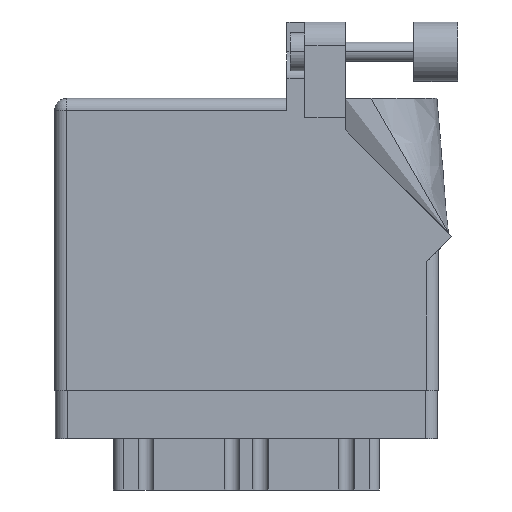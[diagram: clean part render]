
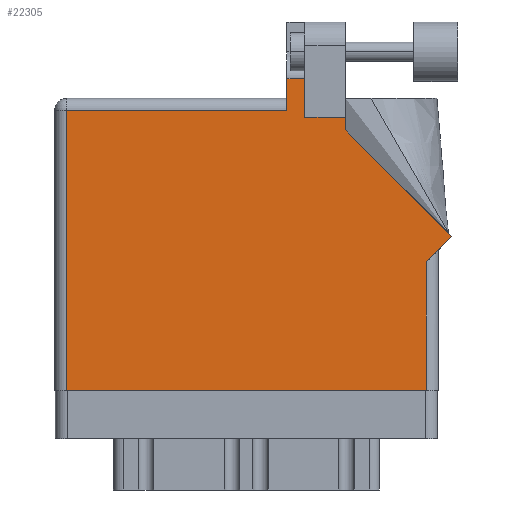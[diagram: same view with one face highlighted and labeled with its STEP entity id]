
A CAD part, front view. The second image highlights one B-rep face of the part: STEP entity #22305.
In plain terms, the highlighted face is planar.
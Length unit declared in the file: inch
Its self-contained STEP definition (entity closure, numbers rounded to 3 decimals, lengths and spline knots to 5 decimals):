
#768 = VECTOR ( 'NONE', #8616, 39.37008 ) ;
#2090 = VERTEX_POINT ( 'NONE', #25903 ) ;
#2147 = EDGE_CURVE ( 'NONE', #38554, #14837, #14760, .T. ) ;
#3330 = LINE ( 'NONE', #3527, #27098 ) ;
#3527 = CARTESIAN_POINT ( 'NONE',  ( 0., 1.468, 0. ) ) ;
#3662 = CARTESIAN_POINT ( 'NONE',  ( 2.08071, 0.80771, 0. ) ) ;
#3976 = LINE ( 'NONE', #13125, #7910 ) ;
#4213 = CARTESIAN_POINT ( 'NONE',  ( 1.217, 1.53, 0. ) ) ;
#4843 = CARTESIAN_POINT ( 'NONE',  ( 1.524, 1.43, 0. ) ) ;
#5574 = EDGE_CURVE ( 'NONE', #2090, #38554, #28818, .T. ) ;
#5685 = CARTESIAN_POINT ( 'NONE',  ( 1.217, 1.468, 0. ) ) ;
#5913 = VERTEX_POINT ( 'NONE', #30746 ) ;
#5914 = LINE ( 'NONE', #18038, #22443 ) ;
#6269 = EDGE_CURVE ( 'NONE', #5913, #10632, #5914, .T. ) ;
#6902 = CARTESIAN_POINT ( 'NONE',  ( 0., 1.53, 0. ) ) ;
#7211 = LINE ( 'NONE', #4213, #15015 ) ;
#7281 = VERTEX_POINT ( 'NONE', #5685 ) ;
#7496 = PLANE ( 'NONE',  #14637 ) ;
#7572 = CARTESIAN_POINT ( 'NONE',  ( 2.01, 0.737, 0. ) ) ;
#7910 = VECTOR ( 'NONE', #15701, 39.37008 ) ;
#8071 = VERTEX_POINT ( 'NONE', #10970 ) ;
#8616 = DIRECTION ( 'NONE',  ( -0.707, 0.707, 0. ) ) ;
#8940 = ORIENTED_EDGE ( 'NONE', *, *, #12325, .T. ) ;
#9541 = DIRECTION ( 'NONE',  ( 0., 1., 0. ) ) ;
#9595 = VECTOR ( 'NONE', #26621, 39.37008 ) ;
#10022 = CARTESIAN_POINT ( 'NONE',  ( 0.062, 1.468, 0. ) ) ;
#10236 = EDGE_CURVE ( 'NONE', #7281, #25590, #3330, .T. ) ;
#10632 = VERTEX_POINT ( 'NONE', #24888 ) ;
#10731 = EDGE_CURVE ( 'NONE', #10632, #7281, #7211, .T. ) ;
#10733 = VECTOR ( 'NONE', #31941, 39.37008 ) ;
#10970 = CARTESIAN_POINT ( 'NONE',  ( 1.311, 1.43, 0. ) ) ;
#12235 = LINE ( 'NONE', #20640, #21302 ) ;
#12325 = EDGE_CURVE ( 'NONE', #35498, #21188, #3976, .T. ) ;
#13125 = CARTESIAN_POINT ( 'NONE',  ( 0., 0., 0. ) ) ;
#13249 = FACE_OUTER_BOUND ( 'NONE', #18243, .T. ) ;
#13968 = LINE ( 'NONE', #4843, #37561 ) ;
#14188 = CARTESIAN_POINT ( 'NONE',  ( 1.948, 0., 0. ) ) ;
#14637 = AXIS2_PLACEMENT_3D ( 'NONE', #6902, #28750, #31706 ) ;
#14760 = LINE ( 'NONE', #23521, #768 ) ;
#14837 = VERTEX_POINT ( 'NONE', #35404 ) ;
#15015 = VECTOR ( 'NONE', #16342, 39.37008 ) ;
#15212 = EDGE_CURVE ( 'NONE', #21188, #2090, #12235, .T. ) ;
#15701 = DIRECTION ( 'NONE',  ( 1., 0., 0. ) ) ;
#16342 = DIRECTION ( 'NONE',  ( 0., -1., 0. ) ) ;
#18038 = CARTESIAN_POINT ( 'NONE',  ( 1.64177, 1.6315, 0. ) ) ;
#18243 = EDGE_LOOP ( 'NONE', ( #22854, #23946, #32418, #27637, #36050, #8940, #38535, #32536, #32237, #30700, #28570 ) ) ;
#19910 = EDGE_CURVE ( 'NONE', #25590, #35498, #22548, .T. ) ;
#20156 = CARTESIAN_POINT ( 'NONE',  ( 0.062, 0., 0. ) ) ;
#20640 = CARTESIAN_POINT ( 'NONE',  ( 1.948, 0.737, 0. ) ) ;
#20993 = VERTEX_POINT ( 'NONE', #35005 ) ;
#21188 = VERTEX_POINT ( 'NONE', #14188 ) ;
#21302 = VECTOR ( 'NONE', #29577, 39.37008 ) ;
#22305 = ADVANCED_FACE ( 'NONE', ( #13249 ), #7496, .F. ) ;
#22443 = VECTOR ( 'NONE', #30125, 39.37008 ) ;
#22548 = LINE ( 'NONE', #20156, #33516 ) ;
#22827 = CARTESIAN_POINT ( 'NONE',  ( 1.524, 1.36442, 0. ) ) ;
#22854 = ORIENTED_EDGE ( 'NONE', *, *, #34489, .T. ) ;
#23521 = CARTESIAN_POINT ( 'NONE',  ( 2.08071, 0.80771, 0. ) ) ;
#23946 = ORIENTED_EDGE ( 'NONE', *, *, #6269, .T. ) ;
#24625 = CARTESIAN_POINT ( 'NONE',  ( 0.062, 0., 0. ) ) ;
#24642 = CARTESIAN_POINT ( 'NONE',  ( 1.311, 1.43, 0. ) ) ;
#24833 = LINE ( 'NONE', #24642, #35322 ) ;
#24888 = CARTESIAN_POINT ( 'NONE',  ( 1.217, 1.6315, 0. ) ) ;
#25590 = VERTEX_POINT ( 'NONE', #10022 ) ;
#25903 = CARTESIAN_POINT ( 'NONE',  ( 1.948, 0.675, 0. ) ) ;
#26621 = DIRECTION ( 'NONE',  ( 0.707, 0.707, 0. ) ) ;
#27025 = DIRECTION ( 'NONE',  ( -1., 0., 0. ) ) ;
#27098 = VECTOR ( 'NONE', #31131, 39.37008 ) ;
#27637 = ORIENTED_EDGE ( 'NONE', *, *, #10236, .T. ) ;
#28200 = EDGE_CURVE ( 'NONE', #20993, #8071, #13968, .T. ) ;
#28570 = ORIENTED_EDGE ( 'NONE', *, *, #28200, .T. ) ;
#28750 = DIRECTION ( 'NONE',  ( 0., 0., -1. ) ) ;
#28786 = LINE ( 'NONE', #22827, #10733 ) ;
#28818 = LINE ( 'NONE', #7572, #9595 ) ;
#29577 = DIRECTION ( 'NONE',  ( 0., 1., 0. ) ) ;
#30125 = DIRECTION ( 'NONE',  ( -1., 0., 0. ) ) ;
#30700 = ORIENTED_EDGE ( 'NONE', *, *, #36528, .T. ) ;
#30746 = CARTESIAN_POINT ( 'NONE',  ( 1.311, 1.6315, 0. ) ) ;
#31131 = DIRECTION ( 'NONE',  ( -1., 0., 0. ) ) ;
#31706 = DIRECTION ( 'NONE',  ( -1., 0., 0. ) ) ;
#31941 = DIRECTION ( 'NONE',  ( 0., 1., 0. ) ) ;
#32237 = ORIENTED_EDGE ( 'NONE', *, *, #2147, .T. ) ;
#32418 = ORIENTED_EDGE ( 'NONE', *, *, #10731, .T. ) ;
#32536 = ORIENTED_EDGE ( 'NONE', *, *, #5574, .T. ) ;
#33516 = VECTOR ( 'NONE', #37395, 39.37008 ) ;
#34489 = EDGE_CURVE ( 'NONE', #8071, #5913, #24833, .T. ) ;
#35005 = CARTESIAN_POINT ( 'NONE',  ( 1.524, 1.43, 0. ) ) ;
#35322 = VECTOR ( 'NONE', #9541, 39.37008 ) ;
#35404 = CARTESIAN_POINT ( 'NONE',  ( 1.524, 1.36442, 0. ) ) ;
#35498 = VERTEX_POINT ( 'NONE', #24625 ) ;
#36050 = ORIENTED_EDGE ( 'NONE', *, *, #19910, .T. ) ;
#36528 = EDGE_CURVE ( 'NONE', #14837, #20993, #28786, .T. ) ;
#37395 = DIRECTION ( 'NONE',  ( 0., -1., 0. ) ) ;
#37561 = VECTOR ( 'NONE', #27025, 39.37008 ) ;
#38535 = ORIENTED_EDGE ( 'NONE', *, *, #15212, .T. ) ;
#38554 = VERTEX_POINT ( 'NONE', #3662 ) ;
